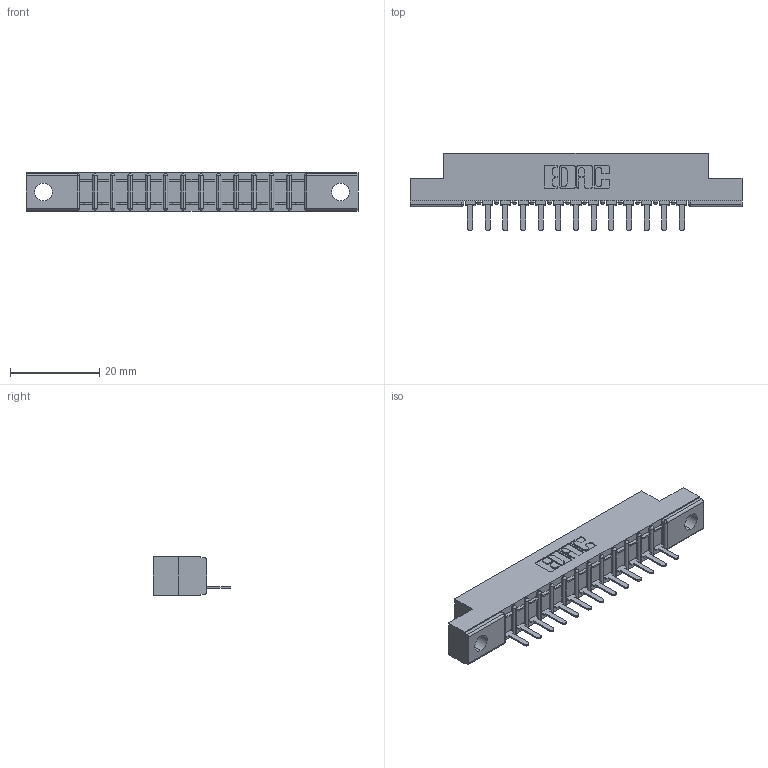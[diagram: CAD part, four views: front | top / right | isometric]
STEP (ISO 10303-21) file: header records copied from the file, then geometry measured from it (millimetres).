
FILE_DESCRIPTION (( 'STEP AP203' ), '1' );
FILE_NAME ('307-013-421-104.STEP', '2020-09-25T13:49:03', ( '' ), ( '' ), 'SwSTEP 2.0', 'SolidWorks 2020', '' );
FILE_SCHEMA (( 'CONFIG_CONTROL_DESIGN' ));
Length unit declared in the file: inch
Products named in the file (3): 307-290-002_521; 307-013-421-104; 307 Part_.156 Dia Mounting Holes
Assembly tree (14 placements, depth 2):
  307-013-421-104
    307 Part_.156 Dia Mounting Holes
    307-290-002_521  x13
Bounding box: 74.52 x 17.42 x 8.71 mm (x, y, z)
Volume: 4810 mm3; surface area: 8146.7 mm2
Topology: 14 solids, 14 shells, 1108 faces, 3375 edges, 2210 vertices
Faces by surface type: plane 669, cylinder 411, sphere 28
Entity records: 15856 total; most frequent: CARTESIAN_POINT 2674, ORIENTED_EDGE 2662, DIRECTION 2603, EDGE_CURVE 1331, LINE 1013, VECTOR 1013, VERTEX_POINT 866, AXIS2_PLACEMENT_3D 795
